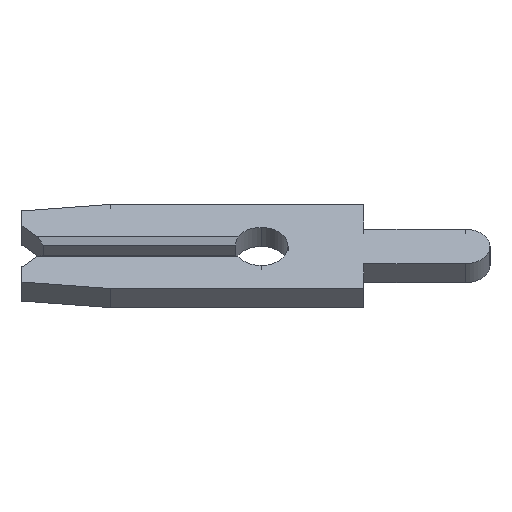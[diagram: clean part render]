
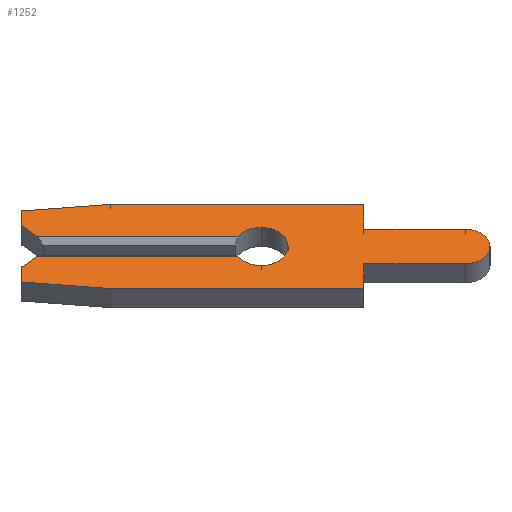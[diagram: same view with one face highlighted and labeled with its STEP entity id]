
A CAD part, left-side view. The second image highlights one B-rep face of the part: STEP entity #1252.
In plain terms, the highlighted face is planar.
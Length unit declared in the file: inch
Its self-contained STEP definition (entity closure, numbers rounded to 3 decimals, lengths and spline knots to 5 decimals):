
#5 = DIRECTION ( 'NONE',  ( 0., -0.707, 0.707 ) ) ;
#12 = DIRECTION ( 'NONE',  ( 0., 0., 1. ) ) ;
#15 = VECTOR ( 'NONE', #12, 39.37008 ) ;
#23 = ORIENTED_EDGE ( 'NONE', *, *, #570, .F. ) ;
#31 = DIRECTION ( 'NONE',  ( 0., 0.707, 0.707 ) ) ;
#45 = LINE ( 'NONE', #1215, #1077 ) ;
#50 = VERTEX_POINT ( 'NONE', #602 ) ;
#53 = EDGE_CURVE ( 'NONE', #1183, #563, #45, .T. ) ;
#60 = DIRECTION ( 'NONE',  ( 0., -0.995, 0.105 ) ) ;
#65 = CARTESIAN_POINT ( 'NONE',  ( -0.013, 0., 0.026 ) ) ;
#68 = LINE ( 'NONE', #622, #349 ) ;
#73 = EDGE_CURVE ( 'NONE', #88, #582, #1134, .T. ) ;
#78 = CARTESIAN_POINT ( 'NONE',  ( -0.013, 0.231, -0.04857 ) ) ;
#88 = VERTEX_POINT ( 'NONE', #105 ) ;
#96 = ORIENTED_EDGE ( 'NONE', *, *, #592, .F. ) ;
#105 = CARTESIAN_POINT ( 'NONE',  ( -0.013, 0.146, -0.0575 ) ) ;
#110 = CARTESIAN_POINT ( 'NONE',  ( -0.013, 0.231, -0.04857 ) ) ;
#113 = VECTOR ( 'NONE', #31, 39.37008 ) ;
#135 = DIRECTION ( 'NONE',  ( -1., 0., 0. ) ) ;
#138 = DIRECTION ( 'NONE',  ( -1., 0., 0. ) ) ;
#157 = ORIENTED_EDGE ( 'NONE', *, *, #732, .T. ) ;
#164 = DIRECTION ( 'NONE',  ( 0., -1., 0. ) ) ;
#176 = CARTESIAN_POINT ( 'NONE',  ( -0.013, 0.231, 0.04857 ) ) ;
#178 = AXIS2_PLACEMENT_3D ( 'NONE', #757, #135, #241 ) ;
#179 = CIRCLE ( 'NONE', #938, 0.026 ) ;
#196 = CARTESIAN_POINT ( 'NONE',  ( -0.013, 0., 0. ) ) ;
#205 = VERTEX_POINT ( 'NONE', #644 ) ;
#221 = CARTESIAN_POINT ( 'NONE',  ( -0.013, -0.099, 0.0235 ) ) ;
#225 = CARTESIAN_POINT ( 'NONE',  ( -0.013, 0.216, -0.013 ) ) ;
#234 = DIRECTION ( 'NONE',  ( 0., 0., -1. ) ) ;
#235 = CARTESIAN_POINT ( 'NONE',  ( -0.013, 0., 0. ) ) ;
#241 = DIRECTION ( 'NONE',  ( 0., 0., -1. ) ) ;
#243 = CARTESIAN_POINT ( 'NONE',  ( -0.013, 0.02252, 0.013 ) ) ;
#263 = LINE ( 'NONE', #176, #917 ) ;
#264 = EDGE_CURVE ( 'NONE', #1191, #1183, #1153, .T. ) ;
#265 = ORIENTED_EDGE ( 'NONE', *, *, #73, .F. ) ;
#277 = FACE_OUTER_BOUND ( 'NONE', #1104, .T. ) ;
#278 = CARTESIAN_POINT ( 'NONE',  ( -0.013, -0.1975, -0.0235 ) ) ;
#282 = VECTOR ( 'NONE', #763, 39.37008 ) ;
#296 = CARTESIAN_POINT ( 'NONE',  ( -0.013, -0.099, -0.0575 ) ) ;
#313 = VERTEX_POINT ( 'NONE', #225 ) ;
#338 = DIRECTION ( 'NONE',  ( 0., -1., 0. ) ) ;
#342 = VERTEX_POINT ( 'NONE', #243 ) ;
#346 = CARTESIAN_POINT ( 'NONE',  ( -0.013, -0.099, -0.0235 ) ) ;
#349 = VECTOR ( 'NONE', #1223, 39.37008 ) ;
#389 = LINE ( 'NONE', #658, #113 ) ;
#390 = DIRECTION ( 'NONE',  ( 0., 1., 0. ) ) ;
#397 = EDGE_CURVE ( 'NONE', #582, #205, #628, .T. ) ;
#431 = ORIENTED_EDGE ( 'NONE', *, *, #641, .F. ) ;
#432 = VERTEX_POINT ( 'NONE', #537 ) ;
#443 = DIRECTION ( 'NONE',  ( 0., -1., 0. ) ) ;
#447 = VECTOR ( 'NONE', #5, 39.37008 ) ;
#489 = AXIS2_PLACEMENT_3D ( 'NONE', #545, #1267, #234 ) ;
#498 = ORIENTED_EDGE ( 'NONE', *, *, #754, .F. ) ;
#506 = DIRECTION ( 'NONE',  ( 1., 0., 0. ) ) ;
#516 = PLANE ( 'NONE',  #677 ) ;
#527 = ORIENTED_EDGE ( 'NONE', *, *, #1110, .F. ) ;
#532 = CARTESIAN_POINT ( 'NONE',  ( -0.013, 0.2105, -0.0075 ) ) ;
#537 = CARTESIAN_POINT ( 'NONE',  ( -0.013, 0.02252, -0.013 ) ) ;
#539 = CARTESIAN_POINT ( 'NONE',  ( -0.013, 0.231, 0.04857 ) ) ;
#545 = CARTESIAN_POINT ( 'NONE',  ( -0.013, 0., 0. ) ) ;
#563 = VERTEX_POINT ( 'NONE', #296 ) ;
#565 = VECTOR ( 'NONE', #935, 39.37008 ) ;
#570 = EDGE_CURVE ( 'NONE', #313, #432, #68, .T. ) ;
#572 = LINE ( 'NONE', #532, #447 ) ;
#581 = AXIS2_PLACEMENT_3D ( 'NONE', #1309, #506, #708 ) ;
#582 = VERTEX_POINT ( 'NONE', #78 ) ;
#584 = VECTOR ( 'NONE', #164, 39.37008 ) ;
#592 = EDGE_CURVE ( 'NONE', #617, #822, #1182, .T. ) ;
#602 = CARTESIAN_POINT ( 'NONE',  ( -0.013, 0.146, 0.0575 ) ) ;
#617 = VERTEX_POINT ( 'NONE', #1053 ) ;
#619 = CARTESIAN_POINT ( 'NONE',  ( -0.013, 0., -0.026 ) ) ;
#622 = CARTESIAN_POINT ( 'NONE',  ( -0.013, 0., -0.013 ) ) ;
#624 = ORIENTED_EDGE ( 'NONE', *, *, #1144, .F. ) ;
#628 = LINE ( 'NONE', #1169, #282 ) ;
#641 = EDGE_CURVE ( 'NONE', #205, #313, #572, .T. ) ;
#644 = CARTESIAN_POINT ( 'NONE',  ( -0.013, 0.231, -0.028 ) ) ;
#658 = CARTESIAN_POINT ( 'NONE',  ( -0.013, 0.2105, 0.0075 ) ) ;
#664 = EDGE_CURVE ( 'NONE', #691, #919, #1014, .T. ) ;
#665 = ORIENTED_EDGE ( 'NONE', *, *, #905, .F. ) ;
#674 = EDGE_CURVE ( 'NONE', #432, #1196, #179, .T. ) ;
#677 = AXIS2_PLACEMENT_3D ( 'NONE', #196, #719, #908 ) ;
#683 = EDGE_CURVE ( 'NONE', #1254, #617, #389, .T. ) ;
#684 = VECTOR ( 'NONE', #338, 39.37008 ) ;
#691 = VERTEX_POINT ( 'NONE', #968 ) ;
#708 = DIRECTION ( 'NONE',  ( 0., 0., 1. ) ) ;
#714 = ORIENTED_EDGE ( 'NONE', *, *, #1007, .F. ) ;
#719 = DIRECTION ( 'NONE',  ( 1., 0., 0. ) ) ;
#732 = EDGE_CURVE ( 'NONE', #1254, #342, #1258, .T. ) ;
#747 = CARTESIAN_POINT ( 'NONE',  ( -0.013, 0.231, 0.013 ) ) ;
#754 = EDGE_CURVE ( 'NONE', #1131, #342, #902, .T. ) ;
#757 = CARTESIAN_POINT ( 'NONE',  ( -0.013, 0., 0. ) ) ;
#762 = DIRECTION ( 'NONE',  ( 0., 0., -1. ) ) ;
#763 = DIRECTION ( 'NONE',  ( 0., 0., 1. ) ) ;
#779 = EDGE_CURVE ( 'NONE', #919, #1020, #1219, .T. ) ;
#805 = CARTESIAN_POINT ( 'NONE',  ( -0.013, 0.146, -0.0575 ) ) ;
#822 = VERTEX_POINT ( 'NONE', #539 ) ;
#829 = LINE ( 'NONE', #805, #862 ) ;
#848 = CIRCLE ( 'NONE', #178, 0.026 ) ;
#858 = CARTESIAN_POINT ( 'NONE',  ( -0.013, -0.099, 0.0235 ) ) ;
#862 = VECTOR ( 'NONE', #390, 39.37008 ) ;
#880 = VECTOR ( 'NONE', #443, 39.37008 ) ;
#895 = CARTESIAN_POINT ( 'NONE',  ( -0.013, -0.099, -0.0235 ) ) ;
#896 = ORIENTED_EDGE ( 'NONE', *, *, #397, .F. ) ;
#902 = CIRCLE ( 'NONE', #489, 0.026 ) ;
#905 = EDGE_CURVE ( 'NONE', #1196, #1131, #848, .T. ) ;
#908 = DIRECTION ( 'NONE',  ( 0., 0., -1. ) ) ;
#917 = VECTOR ( 'NONE', #60, 39.37008 ) ;
#919 = VERTEX_POINT ( 'NONE', #221 ) ;
#924 = DIRECTION ( 'NONE',  ( 0., 0., -1. ) ) ;
#935 = DIRECTION ( 'NONE',  ( 0., 0.995, 0.105 ) ) ;
#938 = AXIS2_PLACEMENT_3D ( 'NONE', #235, #138, #954 ) ;
#954 = DIRECTION ( 'NONE',  ( 0., 0., -1. ) ) ;
#964 = ORIENTED_EDGE ( 'NONE', *, *, #264, .F. ) ;
#968 = CARTESIAN_POINT ( 'NONE',  ( -0.013, -0.099, 0.0575 ) ) ;
#975 = ORIENTED_EDGE ( 'NONE', *, *, #664, .F. ) ;
#991 = CARTESIAN_POINT ( 'NONE',  ( -0.013, -0.1975, 0.0235 ) ) ;
#1007 = EDGE_CURVE ( 'NONE', #822, #50, #263, .T. ) ;
#1014 = LINE ( 'NONE', #1161, #1108 ) ;
#1020 = VERTEX_POINT ( 'NONE', #991 ) ;
#1022 = VECTOR ( 'NONE', #1246, 39.37008 ) ;
#1032 = LINE ( 'NONE', #1199, #584 ) ;
#1053 = CARTESIAN_POINT ( 'NONE',  ( -0.013, 0.231, 0.028 ) ) ;
#1077 = VECTOR ( 'NONE', #924, 39.37008 ) ;
#1097 = CIRCLE ( 'NONE', #581, 0.0235 ) ;
#1104 = EDGE_LOOP ( 'NONE', ( #157, #498, #665, #1224, #23, #431, #896, #265, #624, #1195, #964, #1160, #1234, #975, #527, #714, #96, #1192 ) ) ;
#1108 = VECTOR ( 'NONE', #762, 39.37008 ) ;
#1110 = EDGE_CURVE ( 'NONE', #50, #691, #1032, .T. ) ;
#1131 = VERTEX_POINT ( 'NONE', #65 ) ;
#1134 = LINE ( 'NONE', #110, #565 ) ;
#1144 = EDGE_CURVE ( 'NONE', #563, #88, #829, .T. ) ;
#1147 = CARTESIAN_POINT ( 'NONE',  ( -0.013, 0.231, 0.028 ) ) ;
#1153 = LINE ( 'NONE', #346, #1022 ) ;
#1160 = ORIENTED_EDGE ( 'NONE', *, *, #1185, .F. ) ;
#1161 = CARTESIAN_POINT ( 'NONE',  ( -0.013, -0.099, 0.0575 ) ) ;
#1169 = CARTESIAN_POINT ( 'NONE',  ( -0.013, 0.231, -0.028 ) ) ;
#1182 = LINE ( 'NONE', #1147, #15 ) ;
#1183 = VERTEX_POINT ( 'NONE', #895 ) ;
#1185 = EDGE_CURVE ( 'NONE', #1020, #1191, #1097, .T. ) ;
#1191 = VERTEX_POINT ( 'NONE', #278 ) ;
#1192 = ORIENTED_EDGE ( 'NONE', *, *, #683, .F. ) ;
#1195 = ORIENTED_EDGE ( 'NONE', *, *, #53, .F. ) ;
#1196 = VERTEX_POINT ( 'NONE', #619 ) ;
#1199 = CARTESIAN_POINT ( 'NONE',  ( -0.013, 0.146, 0.0575 ) ) ;
#1213 = CARTESIAN_POINT ( 'NONE',  ( -0.013, 0.216, 0.013 ) ) ;
#1215 = CARTESIAN_POINT ( 'NONE',  ( -0.013, -0.099, -0.0575 ) ) ;
#1219 = LINE ( 'NONE', #858, #684 ) ;
#1223 = DIRECTION ( 'NONE',  ( 0., -1., 0. ) ) ;
#1224 = ORIENTED_EDGE ( 'NONE', *, *, #674, .F. ) ;
#1234 = ORIENTED_EDGE ( 'NONE', *, *, #779, .F. ) ;
#1246 = DIRECTION ( 'NONE',  ( 0., 1., 0. ) ) ;
#1252 = ADVANCED_FACE ( 'NONE', ( #277 ), #516, .F. ) ;
#1254 = VERTEX_POINT ( 'NONE', #1213 ) ;
#1258 = LINE ( 'NONE', #747, #880 ) ;
#1267 = DIRECTION ( 'NONE',  ( -1., 0., 0. ) ) ;
#1309 = CARTESIAN_POINT ( 'NONE',  ( -0.013, -0.1975, 0. ) ) ;
